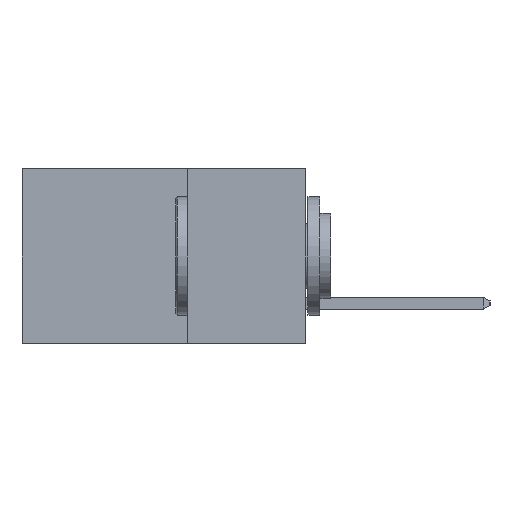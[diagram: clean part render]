
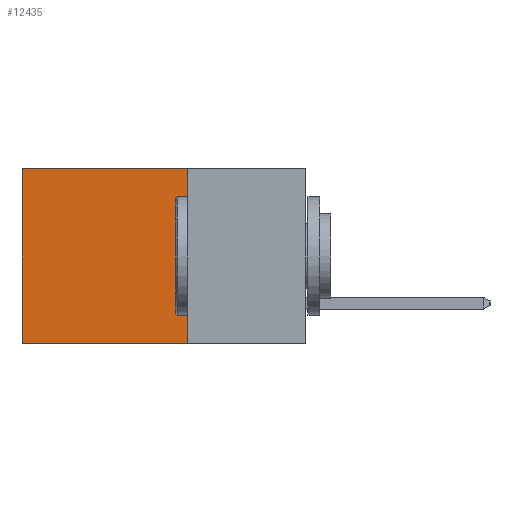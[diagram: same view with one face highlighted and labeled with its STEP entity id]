
A CAD part, left-side view. The second image highlights one B-rep face of the part: STEP entity #12435.
In plain terms, the highlighted planar face has unit normal (-1, 0, 0).
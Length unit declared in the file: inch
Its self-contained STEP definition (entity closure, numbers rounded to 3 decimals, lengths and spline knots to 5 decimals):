
#761 = EDGE_CURVE ( 'NONE', #17357, #5426, #3927, .T. ) ;
#900 = VECTOR ( 'NONE', #14922, 39.37008 ) ;
#1352 = LINE ( 'NONE', #5345, #900 ) ;
#1503 = LINE ( 'NONE', #11698, #8560 ) ;
#1509 = EDGE_LOOP ( 'NONE', ( #16962, #13944, #16844, #4863 ) ) ;
#3157 = CARTESIAN_POINT ( 'NONE',  ( 0.2615, 0.25, -0.37 ) ) ;
#3927 = LINE ( 'NONE', #3157, #17522 ) ;
#4579 = CARTESIAN_POINT ( 'NONE',  ( 0.2615, 0.25, -0.37 ) ) ;
#4589 = EDGE_CURVE ( 'NONE', #8010, #5426, #1352, .T. ) ;
#4863 = ORIENTED_EDGE ( 'NONE', *, *, #11471, .T. ) ;
#5345 = CARTESIAN_POINT ( 'NONE',  ( 0.2615, 0.6, -0.37 ) ) ;
#5426 = VERTEX_POINT ( 'NONE', #12792 ) ;
#5799 = PLANE ( 'NONE',  #10625 ) ;
#5996 = DIRECTION ( 'NONE',  ( 0., 0., -1. ) ) ;
#6019 = FACE_OUTER_BOUND ( 'NONE', #1509, .T. ) ;
#6939 = CARTESIAN_POINT ( 'NONE',  ( 0.2615, 0.6, 0. ) ) ;
#7276 = DIRECTION ( 'NONE',  ( 0., 0., -1. ) ) ;
#8010 = VERTEX_POINT ( 'NONE', #6939 ) ;
#8223 = CARTESIAN_POINT ( 'NONE',  ( 0.2615, 0.25, 0. ) ) ;
#8560 = VECTOR ( 'NONE', #10334, 39.37008 ) ;
#8654 = EDGE_CURVE ( 'NONE', #15458, #17357, #14952, .T. ) ;
#10334 = DIRECTION ( 'NONE',  ( 0., 1., 0. ) ) ;
#10625 = AXIS2_PLACEMENT_3D ( 'NONE', #14052, #15366, #7276 ) ;
#11471 = EDGE_CURVE ( 'NONE', #15458, #8010, #1503, .T. ) ;
#11698 = CARTESIAN_POINT ( 'NONE',  ( 0.2615, 0.25, 0. ) ) ;
#12435 = ADVANCED_FACE ( 'NONE', ( #6019 ), #5799, .F. ) ;
#12792 = CARTESIAN_POINT ( 'NONE',  ( 0.2615, 0.6, -0.37 ) ) ;
#13944 = ORIENTED_EDGE ( 'NONE', *, *, #761, .F. ) ;
#14052 = CARTESIAN_POINT ( 'NONE',  ( 0.2615, 0.25, -0.37 ) ) ;
#14525 = VECTOR ( 'NONE', #5996, 39.37008 ) ;
#14922 = DIRECTION ( 'NONE',  ( 0., 0., -1. ) ) ;
#14952 = LINE ( 'NONE', #4579, #14525 ) ;
#15215 = DIRECTION ( 'NONE',  ( 0., 1., 0. ) ) ;
#15366 = DIRECTION ( 'NONE',  ( 1., 0., 0. ) ) ;
#15458 = VERTEX_POINT ( 'NONE', #8223 ) ;
#16572 = CARTESIAN_POINT ( 'NONE',  ( 0.2615, 0.25, -0.37 ) ) ;
#16844 = ORIENTED_EDGE ( 'NONE', *, *, #8654, .F. ) ;
#16962 = ORIENTED_EDGE ( 'NONE', *, *, #4589, .T. ) ;
#17357 = VERTEX_POINT ( 'NONE', #16572 ) ;
#17522 = VECTOR ( 'NONE', #15215, 39.37008 ) ;
